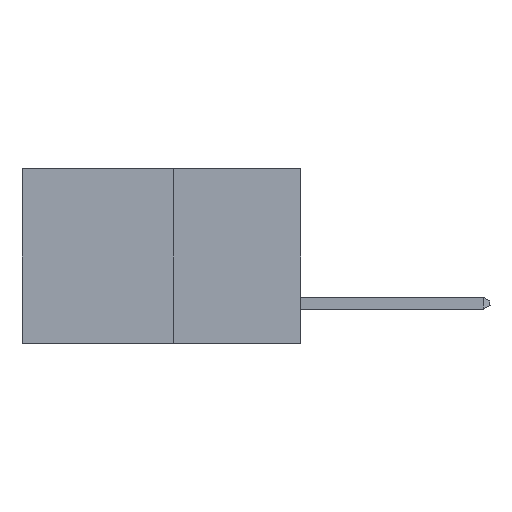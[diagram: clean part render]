
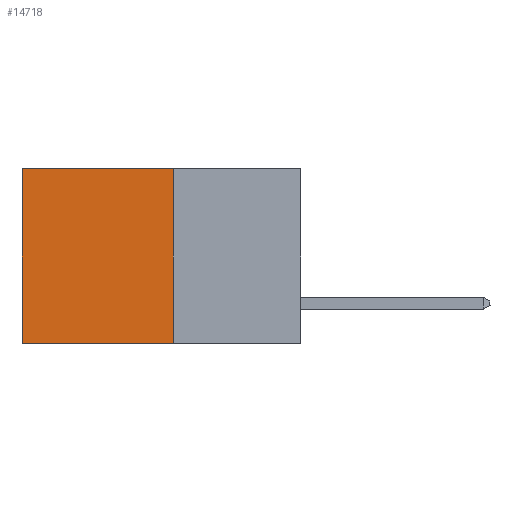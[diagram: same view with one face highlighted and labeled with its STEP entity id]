
A CAD part, left-side view. The second image highlights one B-rep face of the part: STEP entity #14718.
In plain terms, the highlighted planar face has unit normal (-1, 0, 0).
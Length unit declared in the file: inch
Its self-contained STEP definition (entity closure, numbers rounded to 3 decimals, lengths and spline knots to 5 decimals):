
#445 = EDGE_CURVE ( 'NONE', #10480, #15431, #10406, .T. ) ;
#1120 = CARTESIAN_POINT ( 'NONE',  ( 0.277, 0.27, -0.37 ) ) ;
#1712 = DIRECTION ( 'NONE',  ( 0., 0., -1. ) ) ;
#1995 = CARTESIAN_POINT ( 'NONE',  ( 0.277, 0.59, 0. ) ) ;
#2492 = LINE ( 'NONE', #6886, #16320 ) ;
#3706 = FACE_OUTER_BOUND ( 'NONE', #12362, .T. ) ;
#4880 = DIRECTION ( 'NONE',  ( 0., 0., -1. ) ) ;
#5025 = LINE ( 'NONE', #11213, #11381 ) ;
#6143 = ORIENTED_EDGE ( 'NONE', *, *, #445, .T. ) ;
#6245 = EDGE_CURVE ( 'NONE', #8782, #12743, #15256, .T. ) ;
#6886 = CARTESIAN_POINT ( 'NONE',  ( 0.277, 0.59, -0.37 ) ) ;
#7265 = DIRECTION ( 'NONE',  ( 0., 1., 0. ) ) ;
#7440 = DIRECTION ( 'NONE',  ( 0., 1., 0. ) ) ;
#7633 = CARTESIAN_POINT ( 'NONE',  ( 0.277, 0.59, -0.37 ) ) ;
#7681 = EDGE_CURVE ( 'NONE', #15431, #12743, #2492, .T. ) ;
#7797 = ORIENTED_EDGE ( 'NONE', *, *, #7681, .T. ) ;
#7961 = EDGE_CURVE ( 'NONE', #10480, #8782, #5025, .T. ) ;
#8219 = CARTESIAN_POINT ( 'NONE',  ( 0.277, 0.27, -0.37 ) ) ;
#8782 = VERTEX_POINT ( 'NONE', #1120 ) ;
#9484 = CARTESIAN_POINT ( 'NONE',  ( 0.277, 0.27, 0. ) ) ;
#9522 = DIRECTION ( 'NONE',  ( 1., 0., 0. ) ) ;
#9594 = VECTOR ( 'NONE', #7265, 39.37008 ) ;
#10406 = LINE ( 'NONE', #10504, #9594 ) ;
#10480 = VERTEX_POINT ( 'NONE', #9484 ) ;
#10504 = CARTESIAN_POINT ( 'NONE',  ( 0.277, 0.27, 0. ) ) ;
#11042 = ORIENTED_EDGE ( 'NONE', *, *, #7961, .F. ) ;
#11213 = CARTESIAN_POINT ( 'NONE',  ( 0.277, 0.27, -0.37 ) ) ;
#11381 = VECTOR ( 'NONE', #4880, 39.37008 ) ;
#11622 = VECTOR ( 'NONE', #7440, 39.37008 ) ;
#12362 = EDGE_LOOP ( 'NONE', ( #7797, #14020, #11042, #6143 ) ) ;
#12743 = VERTEX_POINT ( 'NONE', #7633 ) ;
#13128 = AXIS2_PLACEMENT_3D ( 'NONE', #8219, #9522, #1712 ) ;
#13752 = CARTESIAN_POINT ( 'NONE',  ( 0.277, 0.27, -0.37 ) ) ;
#14020 = ORIENTED_EDGE ( 'NONE', *, *, #6245, .F. ) ;
#14718 = ADVANCED_FACE ( 'NONE', ( #3706 ), #15704, .F. ) ;
#15256 = LINE ( 'NONE', #13752, #11622 ) ;
#15431 = VERTEX_POINT ( 'NONE', #1995 ) ;
#15604 = DIRECTION ( 'NONE',  ( 0., 0., -1. ) ) ;
#15704 = PLANE ( 'NONE',  #13128 ) ;
#16320 = VECTOR ( 'NONE', #15604, 39.37008 ) ;
